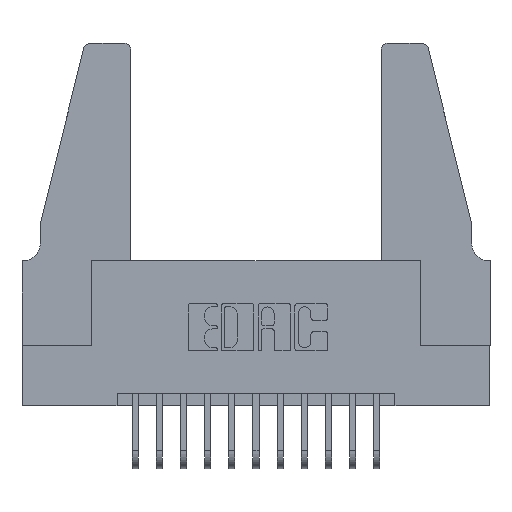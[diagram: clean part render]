
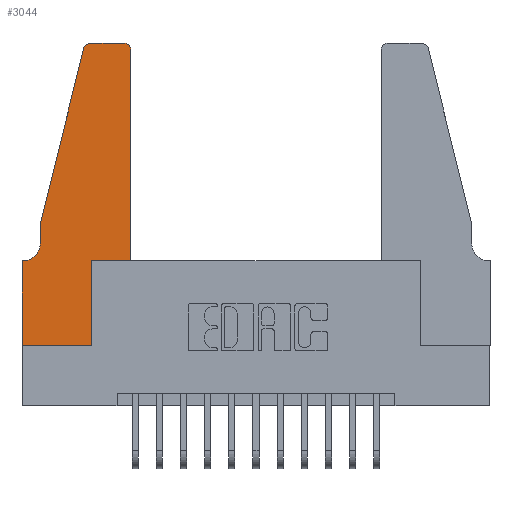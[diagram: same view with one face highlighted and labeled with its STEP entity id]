
A CAD part, top view. The second image highlights one B-rep face of the part: STEP entity #3044.
In plain terms, the highlighted planar face has unit normal (0, 0, 1).
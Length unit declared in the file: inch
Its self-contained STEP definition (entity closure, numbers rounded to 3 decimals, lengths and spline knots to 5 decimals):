
#127 = ORIENTED_EDGE ( 'NONE', *, *, #7163, .T. ) ;
#184 = LINE ( 'NONE', #670, #11988 ) ;
#461 = ORIENTED_EDGE ( 'NONE', *, *, #2330, .T. ) ;
#489 = CARTESIAN_POINT ( 'NONE',  ( 0.4505, 0.35, 0.37 ) ) ;
#604 = ORIENTED_EDGE ( 'NONE', *, *, #3910, .T. ) ;
#670 = CARTESIAN_POINT ( 'NONE',  ( 0.2865, 0.35, 0.37 ) ) ;
#849 = VECTOR ( 'NONE', #2640, 39.37008 ) ;
#1202 = DIRECTION ( 'NONE',  ( 1., 0., 0. ) ) ;
#1219 = EDGE_CURVE ( 'NONE', #13633, #2831, #7334, .T. ) ;
#1323 = VERTEX_POINT ( 'NONE', #8512 ) ;
#1349 = ORIENTED_EDGE ( 'NONE', *, *, #1967, .T. ) ;
#1790 = DIRECTION ( 'NONE',  ( 0., 0., -1. ) ) ;
#1791 = ORIENTED_EDGE ( 'NONE', *, *, #4343, .T. ) ;
#1823 = EDGE_CURVE ( 'NONE', #1323, #11103, #10452, .T. ) ;
#1967 = EDGE_CURVE ( 'NONE', #13531, #1323, #8729, .T. ) ;
#2094 = ORIENTED_EDGE ( 'NONE', *, *, #12982, .T. ) ;
#2330 = EDGE_CURVE ( 'NONE', #8423, #13531, #10436, .T. ) ;
#2466 = CARTESIAN_POINT ( 'NONE',  ( 0.4205, 1.22, 0.37 ) ) ;
#2561 = CARTESIAN_POINT ( 'NONE',  ( 0.0755, 0.5, 0.37 ) ) ;
#2640 = DIRECTION ( 'NONE',  ( -1., 0., 0. ) ) ;
#2831 = VERTEX_POINT ( 'NONE', #10800 ) ;
#2961 = EDGE_CURVE ( 'NONE', #11103, #13564, #4258, .T. ) ;
#3044 = ADVANCED_FACE ( 'NONE', ( #9212 ), #13975, .T. ) ;
#3283 = CARTESIAN_POINT ( 'NONE',  ( 0.0755, 0.5, 0.37 ) ) ;
#3332 = CARTESIAN_POINT ( 'NONE',  ( 0.2865, 0., 0.37 ) ) ;
#3423 = CARTESIAN_POINT ( 'NONE',  ( 0.4505, 0.35, 0.37 ) ) ;
#3790 = CARTESIAN_POINT ( 'NONE',  ( 0.4505, 0.35, 0.37 ) ) ;
#3830 = CIRCLE ( 'NONE', #6703, 0.07 ) ;
#3910 = EDGE_CURVE ( 'NONE', #4786, #9506, #6381, .T. ) ;
#4028 = DIRECTION ( 'NONE',  ( 0., 0., 1. ) ) ;
#4032 = CARTESIAN_POINT ( 'NONE',  ( 0.0755, 0.5, 0.37 ) ) ;
#4089 = AXIS2_PLACEMENT_3D ( 'NONE', #9784, #9757, #13961 ) ;
#4207 = CARTESIAN_POINT ( 'NONE',  ( 0.0755, 0.35, 0.37 ) ) ;
#4258 = CIRCLE ( 'NONE', #12658, 0.03 ) ;
#4322 = CARTESIAN_POINT ( 'NONE',  ( 0.0055, 0.35, 0.37 ) ) ;
#4343 = EDGE_CURVE ( 'NONE', #11993, #10793, #184, .T. ) ;
#4786 = VERTEX_POINT ( 'NONE', #2561 ) ;
#5265 = CARTESIAN_POINT ( 'NONE',  ( 0.4505, 1.22, 0.37 ) ) ;
#5498 = ORIENTED_EDGE ( 'NONE', *, *, #13465, .T. ) ;
#5806 = DIRECTION ( 'NONE',  ( 0., -1., 0. ) ) ;
#5817 = CARTESIAN_POINT ( 'NONE',  ( 0., 0., 0.37 ) ) ;
#6024 = VECTOR ( 'NONE', #8974, 39.37008 ) ;
#6103 = EDGE_CURVE ( 'NONE', #10793, #8423, #7377, .T. ) ;
#6209 = VERTEX_POINT ( 'NONE', #8501 ) ;
#6381 = LINE ( 'NONE', #3283, #6024 ) ;
#6703 = AXIS2_PLACEMENT_3D ( 'NONE', #8653, #1790, #9774 ) ;
#6748 = AXIS2_PLACEMENT_3D ( 'NONE', #2466, #4028, #8485 ) ;
#7163 = EDGE_CURVE ( 'NONE', #6209, #11993, #8204, .T. ) ;
#7334 = LINE ( 'NONE', #4207, #849 ) ;
#7377 = LINE ( 'NONE', #3790, #13322 ) ;
#7466 = CARTESIAN_POINT ( 'NONE',  ( 0.2605, 1.25, 0.37 ) ) ;
#7503 = VECTOR ( 'NONE', #10775, 39.37008 ) ;
#7627 = CARTESIAN_POINT ( 'NONE',  ( 0.25487, 1.22718, 0.37 ) ) ;
#7645 = DIRECTION ( 'NONE',  ( 0., 1., 0. ) ) ;
#7871 = VECTOR ( 'NONE', #1202, 39.37008 ) ;
#7960 = LINE ( 'NONE', #4032, #10562 ) ;
#8003 = LINE ( 'NONE', #12547, #11328 ) ;
#8204 = LINE ( 'NONE', #5817, #7871 ) ;
#8364 = ORIENTED_EDGE ( 'NONE', *, *, #10330, .T. ) ;
#8423 = VERTEX_POINT ( 'NONE', #3423 ) ;
#8485 = DIRECTION ( 'NONE',  ( 1., 0., 0. ) ) ;
#8501 = CARTESIAN_POINT ( 'NONE',  ( 0., 0., 0.37 ) ) ;
#8512 = CARTESIAN_POINT ( 'NONE',  ( 0.4205, 1.25, 0.37 ) ) ;
#8653 = CARTESIAN_POINT ( 'NONE',  ( 0.0055, 0.42, 0.37 ) ) ;
#8705 = DIRECTION ( 'NONE',  ( 0., 1., 0. ) ) ;
#8729 = CIRCLE ( 'NONE', #6748, 0.03 ) ;
#8819 = CARTESIAN_POINT ( 'NONE',  ( 0.284, 1.22, 0.37 ) ) ;
#8933 = DIRECTION ( 'NONE',  ( 0., 0., 1. ) ) ;
#8974 = DIRECTION ( 'NONE',  ( 0., -1., 0. ) ) ;
#9212 = FACE_OUTER_BOUND ( 'NONE', #11555, .T. ) ;
#9506 = VERTEX_POINT ( 'NONE', #9768 ) ;
#9757 = DIRECTION ( 'NONE',  ( 0., 0., 1. ) ) ;
#9768 = CARTESIAN_POINT ( 'NONE',  ( 0.0755, 0.42, 0.37 ) ) ;
#9774 = DIRECTION ( 'NONE',  ( -1., 0., 0. ) ) ;
#9781 = ORIENTED_EDGE ( 'NONE', *, *, #6103, .T. ) ;
#9784 = CARTESIAN_POINT ( 'NONE',  ( 0., 0.35, 0.37 ) ) ;
#10330 = EDGE_CURVE ( 'NONE', #2831, #6209, #8003, .T. ) ;
#10436 = LINE ( 'NONE', #489, #12730 ) ;
#10452 = LINE ( 'NONE', #7466, #7503 ) ;
#10562 = VECTOR ( 'NONE', #13043, 39.37008 ) ;
#10775 = DIRECTION ( 'NONE',  ( -1., 0., 0. ) ) ;
#10778 = CARTESIAN_POINT ( 'NONE',  ( 0.284, 1.25, 0.37 ) ) ;
#10793 = VERTEX_POINT ( 'NONE', #11108 ) ;
#10800 = CARTESIAN_POINT ( 'NONE',  ( 0., 0.35, 0.37 ) ) ;
#10938 = ORIENTED_EDGE ( 'NONE', *, *, #2961, .T. ) ;
#11103 = VERTEX_POINT ( 'NONE', #10778 ) ;
#11108 = CARTESIAN_POINT ( 'NONE',  ( 0.2865, 0.35, 0.37 ) ) ;
#11328 = VECTOR ( 'NONE', #5806, 39.37008 ) ;
#11555 = EDGE_LOOP ( 'NONE', ( #13021, #10938, #5498, #604, #2094, #13275, #8364, #127, #1791, #9781, #461, #1349 ) ) ;
#11675 = DIRECTION ( 'NONE',  ( 1., 0., 0. ) ) ;
#11988 = VECTOR ( 'NONE', #8705, 39.37008 ) ;
#11993 = VERTEX_POINT ( 'NONE', #3332 ) ;
#12547 = CARTESIAN_POINT ( 'NONE',  ( 0., 0., 0.37 ) ) ;
#12658 = AXIS2_PLACEMENT_3D ( 'NONE', #8819, #8933, #14378 ) ;
#12730 = VECTOR ( 'NONE', #7645, 39.37008 ) ;
#12982 = EDGE_CURVE ( 'NONE', #9506, #13633, #3830, .T. ) ;
#13021 = ORIENTED_EDGE ( 'NONE', *, *, #1823, .T. ) ;
#13043 = DIRECTION ( 'NONE',  ( -0.239, -0.971, 0. ) ) ;
#13275 = ORIENTED_EDGE ( 'NONE', *, *, #1219, .T. ) ;
#13322 = VECTOR ( 'NONE', #11675, 39.37008 ) ;
#13465 = EDGE_CURVE ( 'NONE', #13564, #4786, #7960, .T. ) ;
#13531 = VERTEX_POINT ( 'NONE', #5265 ) ;
#13564 = VERTEX_POINT ( 'NONE', #7627 ) ;
#13633 = VERTEX_POINT ( 'NONE', #4322 ) ;
#13961 = DIRECTION ( 'NONE',  ( 1., 0., 0. ) ) ;
#13975 = PLANE ( 'NONE',  #4089 ) ;
#14378 = DIRECTION ( 'NONE',  ( 1., 0., 0. ) ) ;
